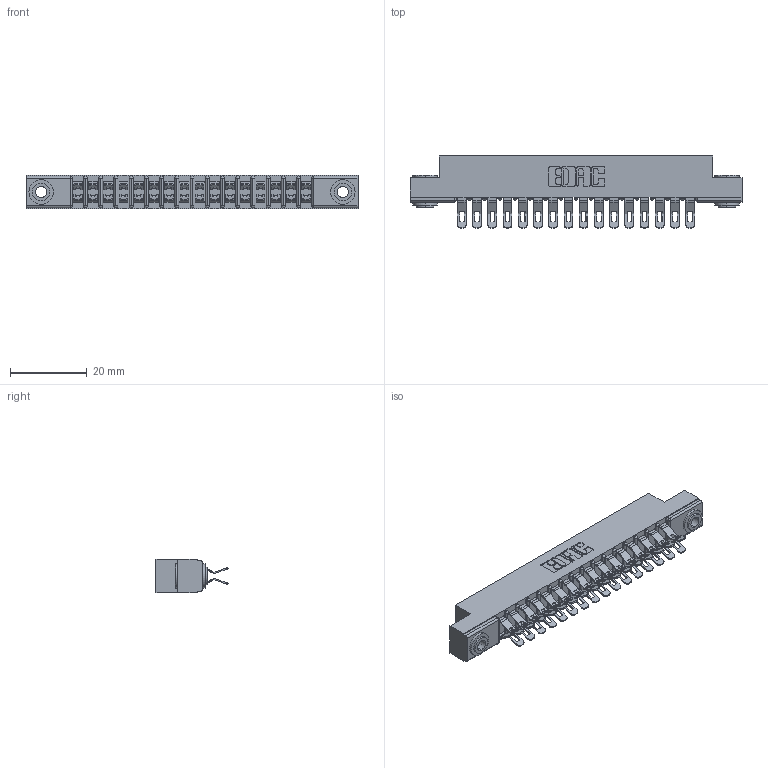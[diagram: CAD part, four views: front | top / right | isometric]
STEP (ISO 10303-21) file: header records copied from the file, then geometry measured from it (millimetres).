
FILE_DESCRIPTION (( 'STEP AP203' ), '1' );
FILE_NAME ('357-032-455-203.STEP', '2020-10-03T14:54:21', ( '' ), ( '' ), 'SwSTEP 2.0', 'SolidWorks 2020', '' );
FILE_SCHEMA (( 'CONFIG_CONTROL_DESIGN' ));
Length unit declared in the file: inch
Products named in the file (4): 307-290-001_555; 345-250-002_345-250-002-102; 307 Part_.156 Dia Mounting Holes; 357-032-455-203
Assembly tree (35 placements, depth 2):
  357-032-455-203
    307 Part_.156 Dia Mounting Holes
    307-290-001_555  x32
    345-250-002_345-250-002-102  x2
Bounding box: 86.41 x 18.75 x 8.71 mm (x, y, z)
Volume: 5749.5 mm3; surface area: 10616 mm2
Topology: 35 solids, 35 shells, 2139 faces, 6227 edges, 4058 vertices
Faces by surface type: plane 1182, cylinder 915, sphere 34, cone 8
Entity records: 19036 total; most frequent: CARTESIAN_POINT 3109, DIRECTION 3078, ORIENTED_EDGE 3072, EDGE_CURVE 1536, VECTOR 1148, LINE 1148, VERTEX_POINT 996, AXIS2_PLACEMENT_3D 965
